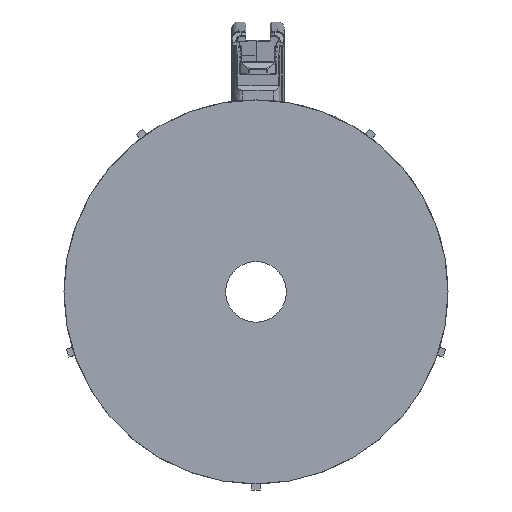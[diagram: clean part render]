
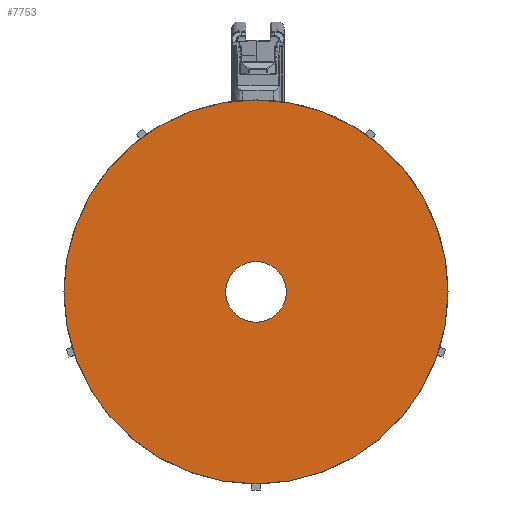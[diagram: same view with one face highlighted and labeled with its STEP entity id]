
A CAD part, front view. The second image highlights one B-rep face of the part: STEP entity #7753.
In plain terms, the highlighted planar face has unit normal (0, -1, 0).
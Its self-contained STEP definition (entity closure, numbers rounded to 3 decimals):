
#574 = FACE_BOUND ( 'NONE', #1197, .T. ) ;
#1190 = CIRCLE ( 'NONE', #2453, 15. ) ;
#1197 = EDGE_LOOP ( 'NONE', ( #4224, #5807 ) ) ;
#1928 = CARTESIAN_POINT ( 'NONE',  ( 0., 0., 95. ) ) ;
#1933 = VERTEX_POINT ( 'NONE', #10586 ) ;
#1936 = EDGE_LOOP ( 'NONE', ( #9930, #7008 ) ) ;
#2390 = CARTESIAN_POINT ( 'NONE',  ( 0., 0., 15. ) ) ;
#2453 = AXIS2_PLACEMENT_3D ( 'NONE', #13955, #6631, #15177 ) ;
#2866 = VERTEX_POINT ( 'NONE', #2390 ) ;
#3266 = CARTESIAN_POINT ( 'NONE',  ( 0., 0., 0. ) ) ;
#3305 = EDGE_CURVE ( 'NONE', #9508, #11967, #5483, .T. ) ;
#3806 = FACE_OUTER_BOUND ( 'NONE', #1936, .T. ) ;
#4212 = DIRECTION ( 'NONE',  ( 0., 0., 1. ) ) ;
#4224 = ORIENTED_EDGE ( 'NONE', *, *, #4931, .T. ) ;
#4487 = DIRECTION ( 'NONE',  ( 0., 0., 1. ) ) ;
#4906 = EDGE_CURVE ( 'NONE', #2866, #1933, #10909, .T. ) ;
#4931 = EDGE_CURVE ( 'NONE', #1933, #2866, #1190, .T. ) ;
#5483 = CIRCLE ( 'NONE', #7310, 95. ) ;
#5486 = EDGE_CURVE ( 'NONE', #11967, #9508, #8196, .T. ) ;
#5807 = ORIENTED_EDGE ( 'NONE', *, *, #4906, .T. ) ;
#6631 = DIRECTION ( 'NONE',  ( 0., 1., 0. ) ) ;
#6981 = CARTESIAN_POINT ( 'NONE',  ( 0., 0., 0. ) ) ;
#7008 = ORIENTED_EDGE ( 'NONE', *, *, #3305, .F. ) ;
#7269 = DIRECTION ( 'NONE',  ( 0., 1., 0. ) ) ;
#7310 = AXIS2_PLACEMENT_3D ( 'NONE', #6981, #15519, #8224 ) ;
#7753 = ADVANCED_FACE ( 'NONE', ( #3806, #574 ), #7840, .F. ) ;
#7840 = PLANE ( 'NONE',  #11980 ) ;
#8196 = CIRCLE ( 'NONE', #11139, 95. ) ;
#8224 = DIRECTION ( 'NONE',  ( 0., 0., 1. ) ) ;
#9508 = VERTEX_POINT ( 'NONE', #1928 ) ;
#9930 = ORIENTED_EDGE ( 'NONE', *, *, #5486, .F. ) ;
#10290 = CARTESIAN_POINT ( 'NONE',  ( 0., 0., 0. ) ) ;
#10586 = CARTESIAN_POINT ( 'NONE',  ( 0., 0., -15. ) ) ;
#10909 = CIRCLE ( 'NONE', #14997, 15. ) ;
#11139 = AXIS2_PLACEMENT_3D ( 'NONE', #3266, #11799, #4487 ) ;
#11528 = DIRECTION ( 'NONE',  ( 0., 1., 0. ) ) ;
#11645 = CARTESIAN_POINT ( 'NONE',  ( 0., 0., -95. ) ) ;
#11799 = DIRECTION ( 'NONE',  ( 0., 1., 0. ) ) ;
#11967 = VERTEX_POINT ( 'NONE', #11645 ) ;
#11980 = AXIS2_PLACEMENT_3D ( 'NONE', #10290, #11528, #4212 ) ;
#13955 = CARTESIAN_POINT ( 'NONE',  ( 0., 0., 0. ) ) ;
#14577 = CARTESIAN_POINT ( 'NONE',  ( 0., 0., 0. ) ) ;
#14997 = AXIS2_PLACEMENT_3D ( 'NONE', #14577, #7269, #15794 ) ;
#15177 = DIRECTION ( 'NONE',  ( 0., 0., 1. ) ) ;
#15519 = DIRECTION ( 'NONE',  ( 0., 1., 0. ) ) ;
#15794 = DIRECTION ( 'NONE',  ( 0., 0., 1. ) ) ;
